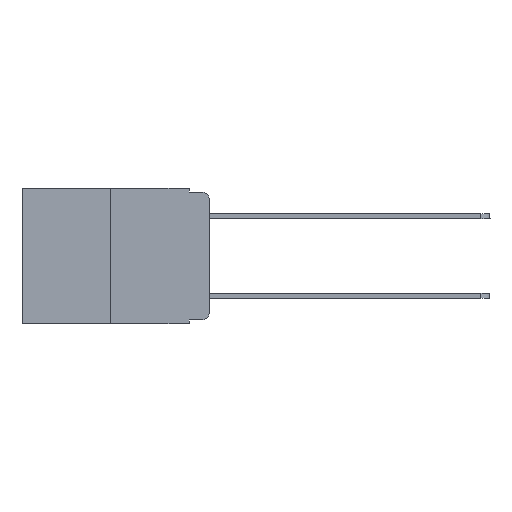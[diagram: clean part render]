
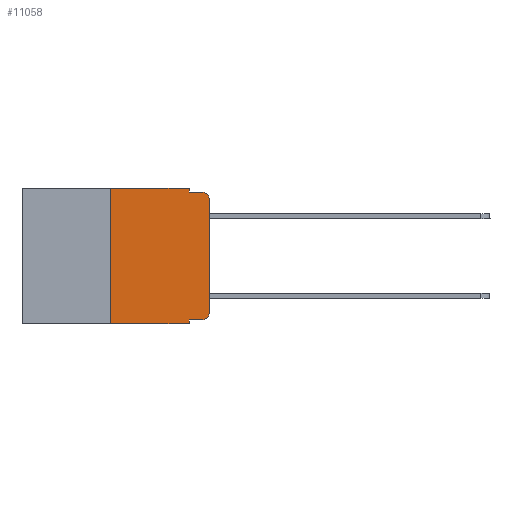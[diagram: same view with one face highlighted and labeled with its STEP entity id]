
A CAD part, left-side view. The second image highlights one B-rep face of the part: STEP entity #11058.
In plain terms, the highlighted planar face has unit normal (-1, 0, 0).
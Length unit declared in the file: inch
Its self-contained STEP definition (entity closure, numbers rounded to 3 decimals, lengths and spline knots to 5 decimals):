
#23 = VERTEX_POINT ( 'NONE', #15830 ) ;
#66 = EDGE_CURVE ( 'NONE', #915, #6305, #9270, .T. ) ;
#112 = EDGE_CURVE ( 'NONE', #2572, #9726, #14708, .T. ) ;
#163 = CARTESIAN_POINT ( 'NONE',  ( 0., 0., -0.03 ) ) ;
#232 = VECTOR ( 'NONE', #570, 39.37008 ) ;
#340 = VECTOR ( 'NONE', #4149, 39.37008 ) ;
#570 = DIRECTION ( 'NONE',  ( 0., -1., 0. ) ) ;
#572 = PLANE ( 'NONE',  #16785 ) ;
#811 = CARTESIAN_POINT ( 'NONE',  ( 0., 0.051, 0. ) ) ;
#915 = VERTEX_POINT ( 'NONE', #16220 ) ;
#953 = AXIS2_PLACEMENT_3D ( 'NONE', #1283, #13358, #6655 ) ;
#1283 = CARTESIAN_POINT ( 'NONE',  ( 0., 0.02, -0.03 ) ) ;
#1855 = VECTOR ( 'NONE', #12829, 39.37008 ) ;
#1856 = EDGE_CURVE ( 'NONE', #15682, #7887, #7772, .T. ) ;
#1932 = CARTESIAN_POINT ( 'NONE',  ( 0., 0.051, -0.333 ) ) ;
#2198 = VERTEX_POINT ( 'NONE', #1932 ) ;
#2540 = VECTOR ( 'NONE', #14145, 39.37008 ) ;
#2572 = VERTEX_POINT ( 'NONE', #3767 ) ;
#2579 = CARTESIAN_POINT ( 'NONE',  ( 0., 0.25, 0. ) ) ;
#3116 = DIRECTION ( 'NONE',  ( 0., 0., -1. ) ) ;
#3177 = EDGE_CURVE ( 'NONE', #2198, #915, #14831, .T. ) ;
#3205 = CARTESIAN_POINT ( 'NONE',  ( 0., 0.02, -0.01 ) ) ;
#3241 = CARTESIAN_POINT ( 'NONE',  ( 0., 0.473, -0.343 ) ) ;
#3313 = EDGE_CURVE ( 'NONE', #23, #15682, #12918, .T. ) ;
#3427 = ORIENTED_EDGE ( 'NONE', *, *, #4883, .T. ) ;
#3657 = LINE ( 'NONE', #5905, #12028 ) ;
#3676 = EDGE_LOOP ( 'NONE', ( #3427, #10790, #7063, #11190, #11540, #14341, #8250, #12517, #12639, #15442 ) ) ;
#3767 = CARTESIAN_POINT ( 'NONE',  ( 0., 0.25, -0.343 ) ) ;
#3954 = VECTOR ( 'NONE', #11874, 39.37008 ) ;
#4149 = DIRECTION ( 'NONE',  ( 0., -1., 0. ) ) ;
#4277 = CARTESIAN_POINT ( 'NONE',  ( 0., 0.051, -0.01 ) ) ;
#4883 = EDGE_CURVE ( 'NONE', #6305, #16794, #3657, .T. ) ;
#5905 = CARTESIAN_POINT ( 'NONE',  ( 0., 0., 0. ) ) ;
#6305 = VERTEX_POINT ( 'NONE', #10130 ) ;
#6655 = DIRECTION ( 'NONE',  ( 0., 0., -1. ) ) ;
#7063 = ORIENTED_EDGE ( 'NONE', *, *, #12325, .F. ) ;
#7552 = LINE ( 'NONE', #7760, #1855 ) ;
#7615 = FACE_OUTER_BOUND ( 'NONE', #3676, .T. ) ;
#7760 = CARTESIAN_POINT ( 'NONE',  ( 0., 0.051, 0. ) ) ;
#7772 = LINE ( 'NONE', #811, #10902 ) ;
#7887 = VERTEX_POINT ( 'NONE', #4277 ) ;
#8039 = CARTESIAN_POINT ( 'NONE',  ( 0., 0.051, -0.343 ) ) ;
#8250 = ORIENTED_EDGE ( 'NONE', *, *, #112, .T. ) ;
#9084 = CARTESIAN_POINT ( 'NONE',  ( 0., 0.473, 0. ) ) ;
#9171 = AXIS2_PLACEMENT_3D ( 'NONE', #11210, #11381, #16552 ) ;
#9270 = CIRCLE ( 'NONE', #9171, 0.02 ) ;
#9461 = VECTOR ( 'NONE', #10610, 39.37008 ) ;
#9726 = VERTEX_POINT ( 'NONE', #8039 ) ;
#9885 = LINE ( 'NONE', #12785, #2540 ) ;
#10130 = CARTESIAN_POINT ( 'NONE',  ( 0., 0., -0.313 ) ) ;
#10532 = CARTESIAN_POINT ( 'NONE',  ( 0., 0.051, -0.333 ) ) ;
#10610 = DIRECTION ( 'NONE',  ( 0., 0., 1. ) ) ;
#10790 = ORIENTED_EDGE ( 'NONE', *, *, #15341, .T. ) ;
#10902 = VECTOR ( 'NONE', #14183, 39.37008 ) ;
#11058 = ADVANCED_FACE ( 'NONE', ( #7615 ), #572, .F. ) ;
#11156 = DIRECTION ( 'NONE',  ( 1., 0., 0. ) ) ;
#11190 = ORIENTED_EDGE ( 'NONE', *, *, #1856, .F. ) ;
#11210 = CARTESIAN_POINT ( 'NONE',  ( 0., 0.02, -0.313 ) ) ;
#11373 = EDGE_CURVE ( 'NONE', #2572, #23, #12581, .T. ) ;
#11381 = DIRECTION ( 'NONE',  ( -1., 0., 0. ) ) ;
#11528 = CARTESIAN_POINT ( 'NONE',  ( 0., 0.051, 0. ) ) ;
#11540 = ORIENTED_EDGE ( 'NONE', *, *, #3313, .F. ) ;
#11874 = DIRECTION ( 'NONE',  ( 0., -1., 0. ) ) ;
#12028 = VECTOR ( 'NONE', #16876, 39.37008 ) ;
#12325 = EDGE_CURVE ( 'NONE', #7887, #14318, #9885, .T. ) ;
#12478 = CARTESIAN_POINT ( 'NONE',  ( 0., 0.473, 0. ) ) ;
#12517 = ORIENTED_EDGE ( 'NONE', *, *, #13335, .F. ) ;
#12581 = LINE ( 'NONE', #2579, #9461 ) ;
#12639 = ORIENTED_EDGE ( 'NONE', *, *, #3177, .T. ) ;
#12785 = CARTESIAN_POINT ( 'NONE',  ( 0., 0.051, -0.01 ) ) ;
#12829 = DIRECTION ( 'NONE',  ( 0., 0., -1. ) ) ;
#12918 = LINE ( 'NONE', #9084, #340 ) ;
#13335 = EDGE_CURVE ( 'NONE', #2198, #9726, #7552, .T. ) ;
#13358 = DIRECTION ( 'NONE',  ( -1., 0., 0. ) ) ;
#14145 = DIRECTION ( 'NONE',  ( 0., -1., 0. ) ) ;
#14183 = DIRECTION ( 'NONE',  ( 0., 0., -1. ) ) ;
#14318 = VERTEX_POINT ( 'NONE', #3205 ) ;
#14341 = ORIENTED_EDGE ( 'NONE', *, *, #11373, .F. ) ;
#14708 = LINE ( 'NONE', #3241, #232 ) ;
#14831 = LINE ( 'NONE', #10532, #3954 ) ;
#15213 = CIRCLE ( 'NONE', #953, 0.02 ) ;
#15341 = EDGE_CURVE ( 'NONE', #16794, #14318, #15213, .T. ) ;
#15442 = ORIENTED_EDGE ( 'NONE', *, *, #66, .T. ) ;
#15682 = VERTEX_POINT ( 'NONE', #11528 ) ;
#15830 = CARTESIAN_POINT ( 'NONE',  ( 0., 0.25, 0. ) ) ;
#16220 = CARTESIAN_POINT ( 'NONE',  ( 0., 0.02, -0.333 ) ) ;
#16552 = DIRECTION ( 'NONE',  ( 0., 0., -1. ) ) ;
#16785 = AXIS2_PLACEMENT_3D ( 'NONE', #12478, #11156, #3116 ) ;
#16794 = VERTEX_POINT ( 'NONE', #163 ) ;
#16876 = DIRECTION ( 'NONE',  ( 0., 0., 1. ) ) ;
